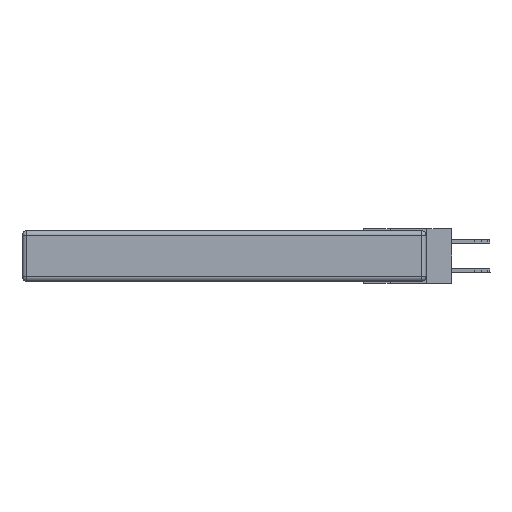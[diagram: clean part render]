
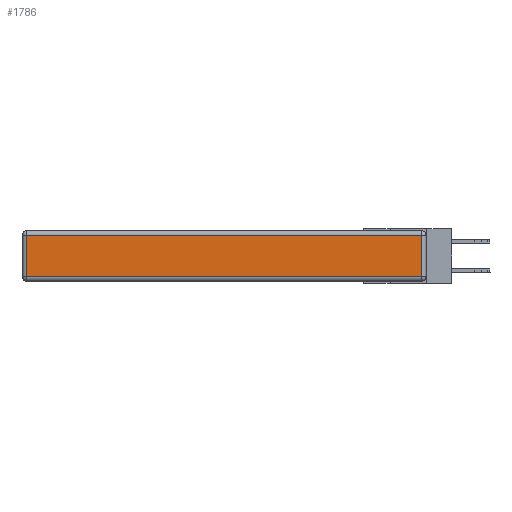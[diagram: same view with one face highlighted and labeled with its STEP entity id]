
A CAD part, left-side view. The second image highlights one B-rep face of the part: STEP entity #1786.
In plain terms, the highlighted planar face has unit normal (-1, 0, 0).
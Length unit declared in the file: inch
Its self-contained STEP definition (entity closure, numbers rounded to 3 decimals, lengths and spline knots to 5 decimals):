
#738 = LINE ( 'NONE', #15492, #7035 ) ;
#1023 = LINE ( 'NONE', #7892, #4407 ) ;
#1367 = VERTEX_POINT ( 'NONE', #8335 ) ;
#1786 = ADVANCED_FACE ( 'NONE', ( #3831 ), #3045, .T. ) ;
#2294 = VERTEX_POINT ( 'NONE', #12724 ) ;
#2626 = LINE ( 'NONE', #8187, #8268 ) ;
#3045 = PLANE ( 'NONE',  #8742 ) ;
#3285 = DIRECTION ( 'NONE',  ( -1., 0., 0. ) ) ;
#3637 = ORIENTED_EDGE ( 'NONE', *, *, #5068, .T. ) ;
#3831 = FACE_OUTER_BOUND ( 'NONE', #14510, .T. ) ;
#4407 = VECTOR ( 'NONE', #5237, 39.37008 ) ;
#4882 = VECTOR ( 'NONE', #17059, 39.37008 ) ;
#5068 = EDGE_CURVE ( 'NONE', #1367, #10506, #1023, .T. ) ;
#5237 = DIRECTION ( 'NONE',  ( 0., 0., 1. ) ) ;
#5422 = ORIENTED_EDGE ( 'NONE', *, *, #17662, .T. ) ;
#7035 = VECTOR ( 'NONE', #18328, 39.37008 ) ;
#7564 = CARTESIAN_POINT ( 'NONE',  ( 0., 0., -0.343 ) ) ;
#7620 = CARTESIAN_POINT ( 'NONE',  ( 0., 0.03, -0.03 ) ) ;
#7892 = CARTESIAN_POINT ( 'NONE',  ( 0., 0.03, -0.343 ) ) ;
#7996 = ORIENTED_EDGE ( 'NONE', *, *, #8185, .T. ) ;
#8172 = EDGE_CURVE ( 'NONE', #10506, #13489, #10955, .T. ) ;
#8185 = EDGE_CURVE ( 'NONE', #13489, #2294, #2626, .T. ) ;
#8187 = CARTESIAN_POINT ( 'NONE',  ( 0., 2.72, -0.343 ) ) ;
#8268 = VECTOR ( 'NONE', #18539, 39.37008 ) ;
#8335 = CARTESIAN_POINT ( 'NONE',  ( 0., 0.03, -0.313 ) ) ;
#8742 = AXIS2_PLACEMENT_3D ( 'NONE', #7564, #3285, #14515 ) ;
#9457 = CARTESIAN_POINT ( 'NONE',  ( 0., 2.75, -0.03 ) ) ;
#10506 = VERTEX_POINT ( 'NONE', #7620 ) ;
#10955 = LINE ( 'NONE', #9457, #4882 ) ;
#12724 = CARTESIAN_POINT ( 'NONE',  ( 0., 2.72, -0.313 ) ) ;
#12826 = ORIENTED_EDGE ( 'NONE', *, *, #8172, .T. ) ;
#13489 = VERTEX_POINT ( 'NONE', #15570 ) ;
#14510 = EDGE_LOOP ( 'NONE', ( #5422, #3637, #12826, #7996 ) ) ;
#14515 = DIRECTION ( 'NONE',  ( 0., 0., 1. ) ) ;
#15492 = CARTESIAN_POINT ( 'NONE',  ( 0., 0., -0.313 ) ) ;
#15570 = CARTESIAN_POINT ( 'NONE',  ( 0., 2.72, -0.03 ) ) ;
#17059 = DIRECTION ( 'NONE',  ( 0., 1., 0. ) ) ;
#17662 = EDGE_CURVE ( 'NONE', #2294, #1367, #738, .T. ) ;
#18328 = DIRECTION ( 'NONE',  ( 0., -1., 0. ) ) ;
#18539 = DIRECTION ( 'NONE',  ( 0., 0., -1. ) ) ;
